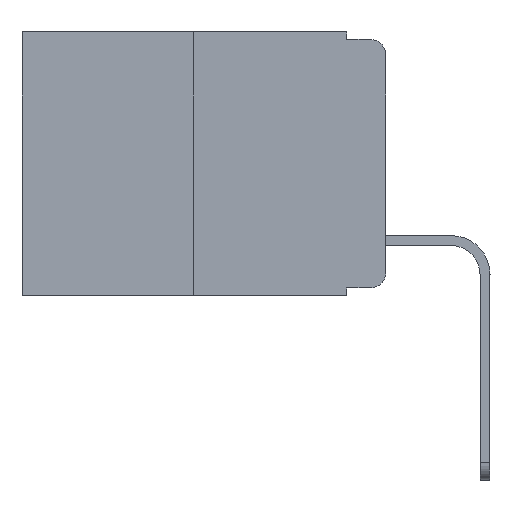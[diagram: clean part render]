
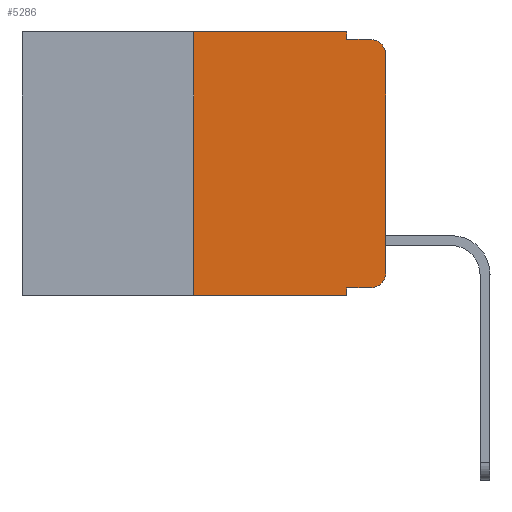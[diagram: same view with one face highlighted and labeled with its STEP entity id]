
A CAD part, left-side view. The second image highlights one B-rep face of the part: STEP entity #5286.
In plain terms, the highlighted planar face has unit normal (-1, 0, 0).
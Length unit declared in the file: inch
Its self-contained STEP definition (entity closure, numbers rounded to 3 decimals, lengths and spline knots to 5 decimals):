
#16 = ORIENTED_EDGE ( 'NONE', *, *, #3313, .F. ) ;
#346 = VERTEX_POINT ( 'NONE', #5610 ) ;
#478 = DIRECTION ( 'NONE',  ( -1., 0., 0. ) ) ;
#553 = ORIENTED_EDGE ( 'NONE', *, *, #13033, .F. ) ;
#698 = DIRECTION ( 'NONE',  ( 0., -1., 0. ) ) ;
#928 = DIRECTION ( 'NONE',  ( 0., 0., -1. ) ) ;
#956 = CARTESIAN_POINT ( 'NONE',  ( 0., 0.051, -0.333 ) ) ;
#1674 = CARTESIAN_POINT ( 'NONE',  ( 0., 0.051, -0.01 ) ) ;
#1750 = CARTESIAN_POINT ( 'NONE',  ( 0., 0.02, -0.313 ) ) ;
#1841 = VECTOR ( 'NONE', #698, 39.37008 ) ;
#2204 = PLANE ( 'NONE',  #11931 ) ;
#2354 = LINE ( 'NONE', #3325, #8663 ) ;
#2498 = LINE ( 'NONE', #5439, #15454 ) ;
#2512 = VERTEX_POINT ( 'NONE', #3335 ) ;
#2853 = DIRECTION ( 'NONE',  ( 0., 0., -1. ) ) ;
#2867 = EDGE_CURVE ( 'NONE', #15191, #12040, #4458, .T. ) ;
#2904 = ORIENTED_EDGE ( 'NONE', *, *, #14969, .F. ) ;
#3107 = LINE ( 'NONE', #3984, #8231 ) ;
#3313 = EDGE_CURVE ( 'NONE', #2512, #12318, #11921, .T. ) ;
#3325 = CARTESIAN_POINT ( 'NONE',  ( 0., 0.25, 0. ) ) ;
#3335 = CARTESIAN_POINT ( 'NONE',  ( 0., 0.051, 0. ) ) ;
#3576 = ORIENTED_EDGE ( 'NONE', *, *, #11576, .T. ) ;
#3954 = AXIS2_PLACEMENT_3D ( 'NONE', #4579, #13311, #5907 ) ;
#3984 = CARTESIAN_POINT ( 'NONE',  ( 0., 0., 0. ) ) ;
#4414 = VECTOR ( 'NONE', #8043, 39.37008 ) ;
#4458 = LINE ( 'NONE', #9156, #9398 ) ;
#4579 = CARTESIAN_POINT ( 'NONE',  ( 0., 0.02, -0.03 ) ) ;
#5182 = EDGE_CURVE ( 'NONE', #15191, #11863, #15008, .T. ) ;
#5286 = ADVANCED_FACE ( 'NONE', ( #11106 ), #2204, .F. ) ;
#5345 = ORIENTED_EDGE ( 'NONE', *, *, #14237, .T. ) ;
#5439 = CARTESIAN_POINT ( 'NONE',  ( 0., 0.473, 0. ) ) ;
#5610 = CARTESIAN_POINT ( 'NONE',  ( 0., 0.02, -0.01 ) ) ;
#5630 = VECTOR ( 'NONE', #11732, 39.37008 ) ;
#5755 = EDGE_CURVE ( 'NONE', #16098, #11863, #14596, .T. ) ;
#5814 = VERTEX_POINT ( 'NONE', #15605 ) ;
#5907 = DIRECTION ( 'NONE',  ( 0., 0., -1. ) ) ;
#5996 = CARTESIAN_POINT ( 'NONE',  ( 0., 0.25, 0. ) ) ;
#7042 = CARTESIAN_POINT ( 'NONE',  ( 0., 0.473, -0.343 ) ) ;
#7172 = CARTESIAN_POINT ( 'NONE',  ( 0., 0.473, 0. ) ) ;
#7516 = EDGE_LOOP ( 'NONE', ( #5345, #9099, #9727, #16, #2904, #553, #12144, #12895, #15015, #3576 ) ) ;
#7649 = VERTEX_POINT ( 'NONE', #10936 ) ;
#8043 = DIRECTION ( 'NONE',  ( 0., 0., -1. ) ) ;
#8231 = VECTOR ( 'NONE', #15099, 39.37008 ) ;
#8663 = VECTOR ( 'NONE', #12060, 39.37008 ) ;
#9099 = ORIENTED_EDGE ( 'NONE', *, *, #10900, .T. ) ;
#9120 = CARTESIAN_POINT ( 'NONE',  ( 0., 0.051, 0. ) ) ;
#9128 = AXIS2_PLACEMENT_3D ( 'NONE', #1750, #478, #2853 ) ;
#9156 = CARTESIAN_POINT ( 'NONE',  ( 0., 0.051, -0.333 ) ) ;
#9371 = CARTESIAN_POINT ( 'NONE',  ( 0., 0.051, -0.01 ) ) ;
#9398 = VECTOR ( 'NONE', #12919, 39.37008 ) ;
#9727 = ORIENTED_EDGE ( 'NONE', *, *, #11673, .F. ) ;
#10900 = EDGE_CURVE ( 'NONE', #5814, #346, #11906, .T. ) ;
#10936 = CARTESIAN_POINT ( 'NONE',  ( 0., 0., -0.313 ) ) ;
#11106 = FACE_OUTER_BOUND ( 'NONE', #7516, .T. ) ;
#11555 = CARTESIAN_POINT ( 'NONE',  ( 0., 0.25, -0.343 ) ) ;
#11576 = EDGE_CURVE ( 'NONE', #12040, #7649, #14243, .T. ) ;
#11673 = EDGE_CURVE ( 'NONE', #12318, #346, #15408, .T. ) ;
#11732 = DIRECTION ( 'NONE',  ( 0., 0., -1. ) ) ;
#11863 = VERTEX_POINT ( 'NONE', #12263 ) ;
#11906 = CIRCLE ( 'NONE', #3954, 0.02 ) ;
#11921 = LINE ( 'NONE', #9120, #5630 ) ;
#11931 = AXIS2_PLACEMENT_3D ( 'NONE', #7172, #15926, #928 ) ;
#12040 = VERTEX_POINT ( 'NONE', #12481 ) ;
#12060 = DIRECTION ( 'NONE',  ( 0., 0., 1. ) ) ;
#12144 = ORIENTED_EDGE ( 'NONE', *, *, #5755, .T. ) ;
#12263 = CARTESIAN_POINT ( 'NONE',  ( 0., 0.051, -0.343 ) ) ;
#12318 = VERTEX_POINT ( 'NONE', #1674 ) ;
#12481 = CARTESIAN_POINT ( 'NONE',  ( 0., 0.02, -0.333 ) ) ;
#12594 = VERTEX_POINT ( 'NONE', #5996 ) ;
#12895 = ORIENTED_EDGE ( 'NONE', *, *, #5182, .F. ) ;
#12919 = DIRECTION ( 'NONE',  ( 0., -1., 0. ) ) ;
#13033 = EDGE_CURVE ( 'NONE', #16098, #12594, #2354, .T. ) ;
#13311 = DIRECTION ( 'NONE',  ( -1., 0., 0. ) ) ;
#13886 = DIRECTION ( 'NONE',  ( 0., -1., 0. ) ) ;
#14237 = EDGE_CURVE ( 'NONE', #7649, #5814, #3107, .T. ) ;
#14243 = CIRCLE ( 'NONE', #9128, 0.02 ) ;
#14351 = CARTESIAN_POINT ( 'NONE',  ( 0., 0.051, 0. ) ) ;
#14596 = LINE ( 'NONE', #7042, #14787 ) ;
#14787 = VECTOR ( 'NONE', #13886, 39.37008 ) ;
#14969 = EDGE_CURVE ( 'NONE', #12594, #2512, #2498, .T. ) ;
#15008 = LINE ( 'NONE', #14351, #4414 ) ;
#15015 = ORIENTED_EDGE ( 'NONE', *, *, #2867, .T. ) ;
#15099 = DIRECTION ( 'NONE',  ( 0., 0., 1. ) ) ;
#15191 = VERTEX_POINT ( 'NONE', #956 ) ;
#15408 = LINE ( 'NONE', #9371, #1841 ) ;
#15454 = VECTOR ( 'NONE', #15457, 39.37008 ) ;
#15457 = DIRECTION ( 'NONE',  ( 0., -1., 0. ) ) ;
#15605 = CARTESIAN_POINT ( 'NONE',  ( 0., 0., -0.03 ) ) ;
#15926 = DIRECTION ( 'NONE',  ( 1., 0., 0. ) ) ;
#16098 = VERTEX_POINT ( 'NONE', #11555 ) ;
